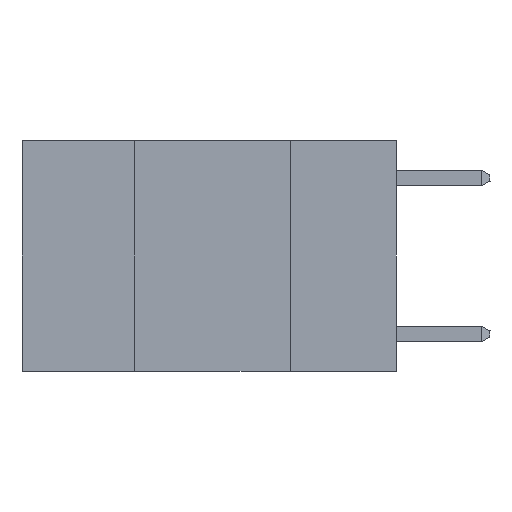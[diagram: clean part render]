
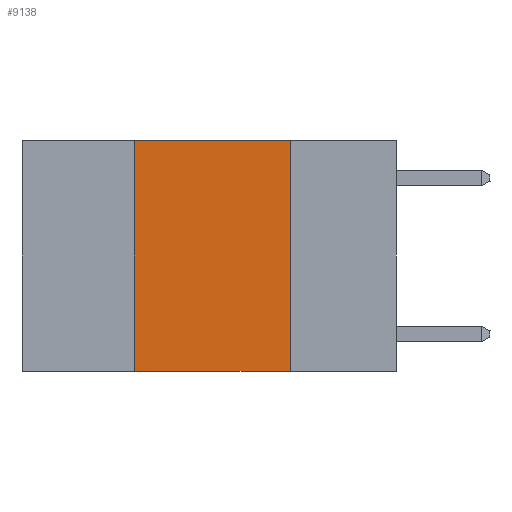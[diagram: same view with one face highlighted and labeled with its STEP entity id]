
A CAD part, left-side view. The second image highlights one B-rep face of the part: STEP entity #9138.
In plain terms, the highlighted planar face has unit normal (-1, 0, 0).
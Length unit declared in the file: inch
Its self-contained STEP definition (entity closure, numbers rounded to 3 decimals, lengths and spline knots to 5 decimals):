
#369 = LINE ( 'NONE', #12777, #5657 ) ;
#1096 = CARTESIAN_POINT ( 'NONE',  ( 0., 0.6, 0. ) ) ;
#1517 = LINE ( 'NONE', #9363, #5695 ) ;
#1779 = EDGE_CURVE ( 'NONE', #5525, #10027, #1517, .T. ) ;
#2332 = DIRECTION ( 'NONE',  ( 0., 0., -1. ) ) ;
#3123 = ORIENTED_EDGE ( 'NONE', *, *, #6403, .F. ) ;
#3333 = DIRECTION ( 'NONE',  ( 0., -1., 0. ) ) ;
#3422 = CARTESIAN_POINT ( 'NONE',  ( 0., 0.6, 0. ) ) ;
#4015 = PLANE ( 'NONE',  #12569 ) ;
#4082 = DIRECTION ( 'NONE',  ( 0., -1., 0. ) ) ;
#4735 = VECTOR ( 'NONE', #2332, 39.37008 ) ;
#5219 = EDGE_CURVE ( 'NONE', #5525, #7418, #369, .T. ) ;
#5324 = LINE ( 'NONE', #3422, #10591 ) ;
#5330 = DIRECTION ( 'NONE',  ( 0., 0., -1. ) ) ;
#5525 = VERTEX_POINT ( 'NONE', #10485 ) ;
#5657 = VECTOR ( 'NONE', #12722, 39.37008 ) ;
#5695 = VECTOR ( 'NONE', #4082, 39.37008 ) ;
#6403 = EDGE_CURVE ( 'NONE', #7418, #9808, #5324, .T. ) ;
#6601 = CARTESIAN_POINT ( 'NONE',  ( 0., 0.17, 0. ) ) ;
#7418 = VERTEX_POINT ( 'NONE', #9941 ) ;
#7585 = LINE ( 'NONE', #6601, #4735 ) ;
#7923 = ORIENTED_EDGE ( 'NONE', *, *, #5219, .F. ) ;
#8640 = ORIENTED_EDGE ( 'NONE', *, *, #10140, .F. ) ;
#9138 = ADVANCED_FACE ( 'NONE', ( #10509 ), #4015, .F. ) ;
#9363 = CARTESIAN_POINT ( 'NONE',  ( 0., 0.6, -0.37 ) ) ;
#9446 = CARTESIAN_POINT ( 'NONE',  ( 0., 0.17, 0. ) ) ;
#9808 = VERTEX_POINT ( 'NONE', #9446 ) ;
#9941 = CARTESIAN_POINT ( 'NONE',  ( 0., 0.42, 0. ) ) ;
#10027 = VERTEX_POINT ( 'NONE', #10595 ) ;
#10140 = EDGE_CURVE ( 'NONE', #9808, #10027, #7585, .T. ) ;
#10485 = CARTESIAN_POINT ( 'NONE',  ( 0., 0.42, -0.37 ) ) ;
#10509 = FACE_OUTER_BOUND ( 'NONE', #10640, .T. ) ;
#10591 = VECTOR ( 'NONE', #3333, 39.37008 ) ;
#10595 = CARTESIAN_POINT ( 'NONE',  ( 0., 0.17, -0.37 ) ) ;
#10640 = EDGE_LOOP ( 'NONE', ( #8640, #3123, #7923, #12932 ) ) ;
#11623 = DIRECTION ( 'NONE',  ( 1., 0., 0. ) ) ;
#12569 = AXIS2_PLACEMENT_3D ( 'NONE', #1096, #11623, #5330 ) ;
#12722 = DIRECTION ( 'NONE',  ( 0., 0., 1. ) ) ;
#12777 = CARTESIAN_POINT ( 'NONE',  ( 0., 0.42, 0. ) ) ;
#12932 = ORIENTED_EDGE ( 'NONE', *, *, #1779, .T. ) ;
